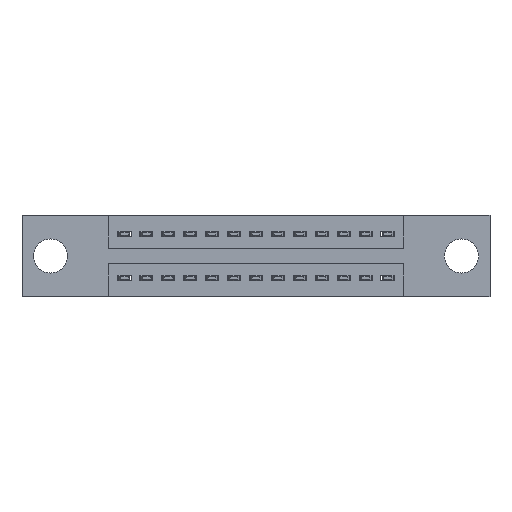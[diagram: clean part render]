
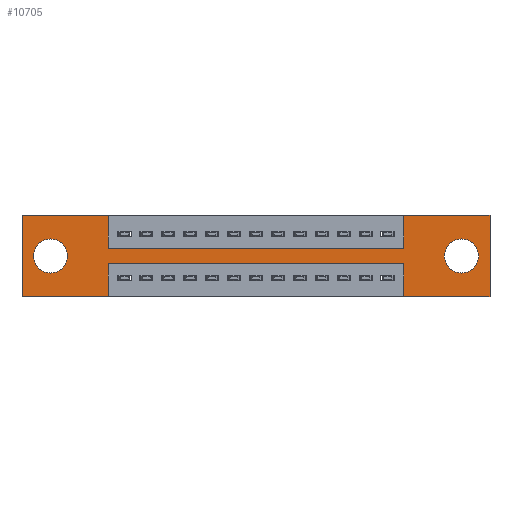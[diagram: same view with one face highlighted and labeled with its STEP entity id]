
A CAD part, front view. The second image highlights one B-rep face of the part: STEP entity #10705.
In plain terms, the highlighted planar face has unit normal (0, -1, 0).
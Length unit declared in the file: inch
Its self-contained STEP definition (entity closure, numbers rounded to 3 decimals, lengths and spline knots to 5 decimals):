
#32 = ORIENTED_EDGE ( 'NONE', *, *, #12887, .T. ) ;
#154 = VERTEX_POINT ( 'NONE', #7468 ) ;
#216 = VECTOR ( 'NONE', #4015, 39.37008 ) ;
#355 = EDGE_LOOP ( 'NONE', ( #5828, #10323, #3791, #4486, #12418, #5320, #7834, #7943, #5027, #5631, #5486, #8010 ) ) ;
#396 = ORIENTED_EDGE ( 'NONE', *, *, #7098, .T. ) ;
#478 = LINE ( 'NONE', #1565, #4190 ) ;
#610 = DIRECTION ( 'NONE',  ( 0., 0., -1. ) ) ;
#737 = CARTESIAN_POINT ( 'NONE',  ( 0., 0., 0. ) ) ;
#740 = CARTESIAN_POINT ( 'NONE',  ( 0., 0., 0. ) ) ;
#804 = LINE ( 'NONE', #737, #6001 ) ;
#805 = LINE ( 'NONE', #877, #9641 ) ;
#877 = CARTESIAN_POINT ( 'NONE',  ( 0.3925, 0., -0.37 ) ) ;
#908 = AXIS2_PLACEMENT_3D ( 'NONE', #2479, #13803, #1600 ) ;
#1014 = VERTEX_POINT ( 'NONE', #2810 ) ;
#1225 = EDGE_CURVE ( 'NONE', #4791, #13189, #9514, .T. ) ;
#1427 = DIRECTION ( 'NONE',  ( 0., 0., 1. ) ) ;
#1499 = LINE ( 'NONE', #3690, #1871 ) ;
#1565 = CARTESIAN_POINT ( 'NONE',  ( 1.7425, 0., 0. ) ) ;
#1600 = DIRECTION ( 'NONE',  ( 0., 0., -1. ) ) ;
#1658 = LINE ( 'NONE', #9418, #13215 ) ;
#1871 = VECTOR ( 'NONE', #10365, 39.37008 ) ;
#2159 = DIRECTION ( 'NONE',  ( 0., -1., 0. ) ) ;
#2312 = CIRCLE ( 'NONE', #908, 0.078 ) ;
#2479 = CARTESIAN_POINT ( 'NONE',  ( 2.005, 0., -0.185 ) ) ;
#2492 = VECTOR ( 'NONE', #11269, 39.37008 ) ;
#2661 = EDGE_CURVE ( 'NONE', #3165, #4791, #11041, .T. ) ;
#2765 = VERTEX_POINT ( 'NONE', #5718 ) ;
#2810 = CARTESIAN_POINT ( 'NONE',  ( 0.13, 0., -0.107 ) ) ;
#2925 = CIRCLE ( 'NONE', #10338, 0.078 ) ;
#2954 = DIRECTION ( 'NONE',  ( 0., 0., 1. ) ) ;
#3099 = VERTEX_POINT ( 'NONE', #13955 ) ;
#3165 = VERTEX_POINT ( 'NONE', #12043 ) ;
#3255 = DIRECTION ( 'NONE',  ( 0., 0., -1. ) ) ;
#3400 = EDGE_CURVE ( 'NONE', #1014, #9354, #2925, .T. ) ;
#3690 = CARTESIAN_POINT ( 'NONE',  ( 0., 0., 0. ) ) ;
#3703 = VECTOR ( 'NONE', #12061, 39.37008 ) ;
#3791 = ORIENTED_EDGE ( 'NONE', *, *, #2661, .F. ) ;
#3898 = EDGE_CURVE ( 'NONE', #9354, #1014, #10993, .T. ) ;
#4015 = DIRECTION ( 'NONE',  ( -1., 0., 0. ) ) ;
#4101 = CARTESIAN_POINT ( 'NONE',  ( 0.13, 0., -0.185 ) ) ;
#4190 = VECTOR ( 'NONE', #2954, 39.37008 ) ;
#4413 = CARTESIAN_POINT ( 'NONE',  ( 0., 0., -0.37 ) ) ;
#4486 = ORIENTED_EDGE ( 'NONE', *, *, #11211, .F. ) ;
#4578 = EDGE_LOOP ( 'NONE', ( #396, #32 ) ) ;
#4738 = AXIS2_PLACEMENT_3D ( 'NONE', #7271, #11714, #9535 ) ;
#4791 = VERTEX_POINT ( 'NONE', #6633 ) ;
#4827 = ORIENTED_EDGE ( 'NONE', *, *, #3400, .T. ) ;
#4901 = VERTEX_POINT ( 'NONE', #5551 ) ;
#4975 = VERTEX_POINT ( 'NONE', #13554 ) ;
#5027 = ORIENTED_EDGE ( 'NONE', *, *, #11961, .F. ) ;
#5048 = CARTESIAN_POINT ( 'NONE',  ( 0.3925, 0., 0. ) ) ;
#5098 = EDGE_CURVE ( 'NONE', #5620, #4975, #478, .T. ) ;
#5238 = CARTESIAN_POINT ( 'NONE',  ( 2.005, 0., -0.185 ) ) ;
#5256 = LINE ( 'NONE', #8515, #7095 ) ;
#5320 = ORIENTED_EDGE ( 'NONE', *, *, #8541, .F. ) ;
#5411 = FACE_OUTER_BOUND ( 'NONE', #355, .T. ) ;
#5486 = ORIENTED_EDGE ( 'NONE', *, *, #12592, .F. ) ;
#5551 = CARTESIAN_POINT ( 'NONE',  ( 2.135, 0., 0. ) ) ;
#5620 = VERTEX_POINT ( 'NONE', #8562 ) ;
#5631 = ORIENTED_EDGE ( 'NONE', *, *, #13333, .F. ) ;
#5718 = CARTESIAN_POINT ( 'NONE',  ( 0.3925, 0., 0. ) ) ;
#5828 = ORIENTED_EDGE ( 'NONE', *, *, #7069, .F. ) ;
#5902 = LINE ( 'NONE', #5048, #11563 ) ;
#6001 = VECTOR ( 'NONE', #11790, 39.37008 ) ;
#6005 = VERTEX_POINT ( 'NONE', #9637 ) ;
#6196 = DIRECTION ( 'NONE',  ( 0., 0., 1. ) ) ;
#6213 = DIRECTION ( 'NONE',  ( 1., 0., 0. ) ) ;
#6331 = DIRECTION ( 'NONE',  ( 0., 1., 0. ) ) ;
#6633 = CARTESIAN_POINT ( 'NONE',  ( 1.7425, 0., -0.22 ) ) ;
#6677 = CARTESIAN_POINT ( 'NONE',  ( 0., 0., 0. ) ) ;
#6969 = DIRECTION ( 'NONE',  ( -1., 0., 0. ) ) ;
#7069 = EDGE_CURVE ( 'NONE', #13189, #6005, #805, .T. ) ;
#7095 = VECTOR ( 'NONE', #7644, 39.37008 ) ;
#7098 = EDGE_CURVE ( 'NONE', #3099, #9872, #7320, .T. ) ;
#7271 = CARTESIAN_POINT ( 'NONE',  ( 0.13, 0., -0.185 ) ) ;
#7320 = CIRCLE ( 'NONE', #10567, 0.078 ) ;
#7421 = DIRECTION ( 'NONE',  ( 0., 0., -1. ) ) ;
#7468 = CARTESIAN_POINT ( 'NONE',  ( 2.135, 0., -0.37 ) ) ;
#7622 = LINE ( 'NONE', #13364, #3703 ) ;
#7644 = DIRECTION ( 'NONE',  ( 0., 0., -1. ) ) ;
#7675 = CARTESIAN_POINT ( 'NONE',  ( 0.3925, 0., -0.15 ) ) ;
#7766 = CARTESIAN_POINT ( 'NONE',  ( 2.005, 0., -0.263 ) ) ;
#7829 = CARTESIAN_POINT ( 'NONE',  ( 1.7425, 0., -0.37 ) ) ;
#7834 = ORIENTED_EDGE ( 'NONE', *, *, #5098, .F. ) ;
#7943 = ORIENTED_EDGE ( 'NONE', *, *, #13532, .F. ) ;
#8010 = ORIENTED_EDGE ( 'NONE', *, *, #11391, .F. ) ;
#8012 = EDGE_CURVE ( 'NONE', #4901, #154, #5256, .T. ) ;
#8515 = CARTESIAN_POINT ( 'NONE',  ( 2.135, 0., 0. ) ) ;
#8537 = CARTESIAN_POINT ( 'NONE',  ( 0., 0., -0.37 ) ) ;
#8541 = EDGE_CURVE ( 'NONE', #4975, #4901, #8866, .T. ) ;
#8546 = AXIS2_PLACEMENT_3D ( 'NONE', #4413, #2159, #3255 ) ;
#8562 = CARTESIAN_POINT ( 'NONE',  ( 1.7425, 0., -0.15 ) ) ;
#8621 = EDGE_LOOP ( 'NONE', ( #4827, #11637 ) ) ;
#8809 = VECTOR ( 'NONE', #1427, 39.37008 ) ;
#8840 = CARTESIAN_POINT ( 'NONE',  ( 0.3925, 0., -0.22 ) ) ;
#8866 = LINE ( 'NONE', #6677, #2492 ) ;
#8940 = VERTEX_POINT ( 'NONE', #7675 ) ;
#8973 = FACE_BOUND ( 'NONE', #4578, .T. ) ;
#9324 = VERTEX_POINT ( 'NONE', #8537 ) ;
#9354 = VERTEX_POINT ( 'NONE', #12842 ) ;
#9418 = CARTESIAN_POINT ( 'NONE',  ( 0.3925, 0., -0.15 ) ) ;
#9514 = LINE ( 'NONE', #12791, #12308 ) ;
#9529 = CARTESIAN_POINT ( 'NONE',  ( 0., 0., -0.37 ) ) ;
#9534 = DIRECTION ( 'NONE',  ( 0., 0., -1. ) ) ;
#9535 = DIRECTION ( 'NONE',  ( 0., 0., 1. ) ) ;
#9637 = CARTESIAN_POINT ( 'NONE',  ( 0.3925, 0., -0.37 ) ) ;
#9641 = VECTOR ( 'NONE', #7421, 39.37008 ) ;
#9872 = VERTEX_POINT ( 'NONE', #7766 ) ;
#10323 = ORIENTED_EDGE ( 'NONE', *, *, #1225, .F. ) ;
#10338 = AXIS2_PLACEMENT_3D ( 'NONE', #4101, #6331, #6196 ) ;
#10365 = DIRECTION ( 'NONE',  ( 1., 0., 0. ) ) ;
#10567 = AXIS2_PLACEMENT_3D ( 'NONE', #5238, #14184, #9534 ) ;
#10612 = LINE ( 'NONE', #9529, #216 ) ;
#10705 = ADVANCED_FACE ( 'NONE', ( #8973, #12249, #5411 ), #12034, .T. ) ;
#10993 = CIRCLE ( 'NONE', #4738, 0.078 ) ;
#11041 = LINE ( 'NONE', #7829, #8809 ) ;
#11211 = EDGE_CURVE ( 'NONE', #154, #3165, #10612, .T. ) ;
#11269 = DIRECTION ( 'NONE',  ( 1., 0., 0. ) ) ;
#11391 = EDGE_CURVE ( 'NONE', #6005, #9324, #7622, .T. ) ;
#11563 = VECTOR ( 'NONE', #610, 39.37008 ) ;
#11637 = ORIENTED_EDGE ( 'NONE', *, *, #3898, .T. ) ;
#11714 = DIRECTION ( 'NONE',  ( 0., 1., 0. ) ) ;
#11790 = DIRECTION ( 'NONE',  ( 0., 0., 1. ) ) ;
#11961 = EDGE_CURVE ( 'NONE', #2765, #8940, #5902, .T. ) ;
#12034 = PLANE ( 'NONE',  #8546 ) ;
#12043 = CARTESIAN_POINT ( 'NONE',  ( 1.7425, 0., -0.37 ) ) ;
#12061 = DIRECTION ( 'NONE',  ( -1., 0., 0. ) ) ;
#12249 = FACE_BOUND ( 'NONE', #8621, .T. ) ;
#12308 = VECTOR ( 'NONE', #6969, 39.37008 ) ;
#12418 = ORIENTED_EDGE ( 'NONE', *, *, #8012, .F. ) ;
#12592 = EDGE_CURVE ( 'NONE', #9324, #13986, #804, .T. ) ;
#12791 = CARTESIAN_POINT ( 'NONE',  ( 0.3925, 0., -0.22 ) ) ;
#12842 = CARTESIAN_POINT ( 'NONE',  ( 0.13, 0., -0.263 ) ) ;
#12887 = EDGE_CURVE ( 'NONE', #9872, #3099, #2312, .T. ) ;
#13189 = VERTEX_POINT ( 'NONE', #8840 ) ;
#13215 = VECTOR ( 'NONE', #6213, 39.37008 ) ;
#13333 = EDGE_CURVE ( 'NONE', #13986, #2765, #1499, .T. ) ;
#13364 = CARTESIAN_POINT ( 'NONE',  ( 0., 0., -0.37 ) ) ;
#13532 = EDGE_CURVE ( 'NONE', #8940, #5620, #1658, .T. ) ;
#13554 = CARTESIAN_POINT ( 'NONE',  ( 1.7425, 0., 0. ) ) ;
#13803 = DIRECTION ( 'NONE',  ( 0., 1., 0. ) ) ;
#13955 = CARTESIAN_POINT ( 'NONE',  ( 2.005, 0., -0.107 ) ) ;
#13986 = VERTEX_POINT ( 'NONE', #740 ) ;
#14184 = DIRECTION ( 'NONE',  ( 0., 1., 0. ) ) ;
